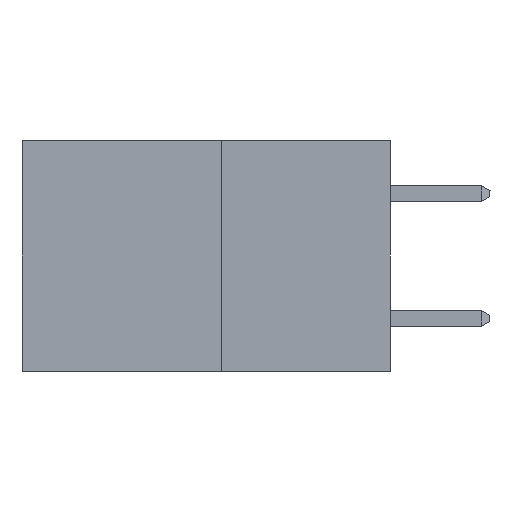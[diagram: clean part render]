
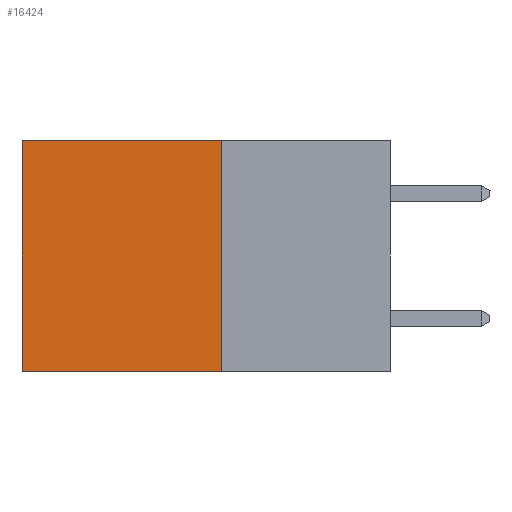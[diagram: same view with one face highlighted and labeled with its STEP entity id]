
A CAD part, left-side view. The second image highlights one B-rep face of the part: STEP entity #16424.
In plain terms, the highlighted planar face has unit normal (-1, 0, 0).
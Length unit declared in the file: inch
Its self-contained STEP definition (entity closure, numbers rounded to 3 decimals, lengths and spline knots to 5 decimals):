
#196 = VECTOR ( 'NONE', #5853, 39.37008 ) ;
#335 = CARTESIAN_POINT ( 'NONE',  ( 0.277, 0.27, 0. ) ) ;
#1408 = CARTESIAN_POINT ( 'NONE',  ( 0.277, 0.59, -0.37 ) ) ;
#1698 = CARTESIAN_POINT ( 'NONE',  ( 0.277, 0.27, -0.37 ) ) ;
#2368 = VECTOR ( 'NONE', #3270, 39.37008 ) ;
#2464 = EDGE_CURVE ( 'NONE', #9614, #9120, #16782, .T. ) ;
#2566 = ORIENTED_EDGE ( 'NONE', *, *, #10765, .F. ) ;
#2855 = LINE ( 'NONE', #1698, #2368 ) ;
#2979 = DIRECTION ( 'NONE',  ( 0., 0., -1. ) ) ;
#3180 = PLANE ( 'NONE',  #10933 ) ;
#3270 = DIRECTION ( 'NONE',  ( 0., 0., -1. ) ) ;
#4802 = LINE ( 'NONE', #10245, #196 ) ;
#4989 = ORIENTED_EDGE ( 'NONE', *, *, #2464, .F. ) ;
#5853 = DIRECTION ( 'NONE',  ( 0., 1., 0. ) ) ;
#6279 = DIRECTION ( 'NONE',  ( 1., 0., 0. ) ) ;
#6575 = VERTEX_POINT ( 'NONE', #9773 ) ;
#7539 = DIRECTION ( 'NONE',  ( 0., 1., 0. ) ) ;
#7924 = LINE ( 'NONE', #1408, #15334 ) ;
#8915 = EDGE_CURVE ( 'NONE', #6575, #9120, #7924, .T. ) ;
#9120 = VERTEX_POINT ( 'NONE', #13895 ) ;
#9614 = VERTEX_POINT ( 'NONE', #15457 ) ;
#9773 = CARTESIAN_POINT ( 'NONE',  ( 0.277, 0.59, 0. ) ) ;
#10245 = CARTESIAN_POINT ( 'NONE',  ( 0.277, 0.27, 0. ) ) ;
#10365 = FACE_OUTER_BOUND ( 'NONE', #16033, .T. ) ;
#10655 = EDGE_CURVE ( 'NONE', #15719, #6575, #4802, .T. ) ;
#10765 = EDGE_CURVE ( 'NONE', #15719, #9614, #2855, .T. ) ;
#10933 = AXIS2_PLACEMENT_3D ( 'NONE', #13649, #6279, #16630 ) ;
#11920 = VECTOR ( 'NONE', #7539, 39.37008 ) ;
#13649 = CARTESIAN_POINT ( 'NONE',  ( 0.277, 0.27, -0.37 ) ) ;
#13895 = CARTESIAN_POINT ( 'NONE',  ( 0.277, 0.59, -0.37 ) ) ;
#14245 = ORIENTED_EDGE ( 'NONE', *, *, #8915, .T. ) ;
#15334 = VECTOR ( 'NONE', #2979, 39.37008 ) ;
#15457 = CARTESIAN_POINT ( 'NONE',  ( 0.277, 0.27, -0.37 ) ) ;
#15719 = VERTEX_POINT ( 'NONE', #335 ) ;
#16033 = EDGE_LOOP ( 'NONE', ( #14245, #4989, #2566, #18161 ) ) ;
#16424 = ADVANCED_FACE ( 'NONE', ( #10365 ), #3180, .F. ) ;
#16630 = DIRECTION ( 'NONE',  ( 0., 0., -1. ) ) ;
#16782 = LINE ( 'NONE', #19271, #11920 ) ;
#18161 = ORIENTED_EDGE ( 'NONE', *, *, #10655, .T. ) ;
#19271 = CARTESIAN_POINT ( 'NONE',  ( 0.277, 0.27, -0.37 ) ) ;
